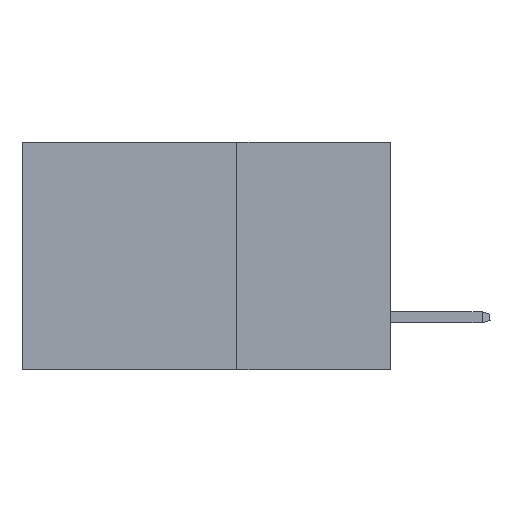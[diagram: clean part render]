
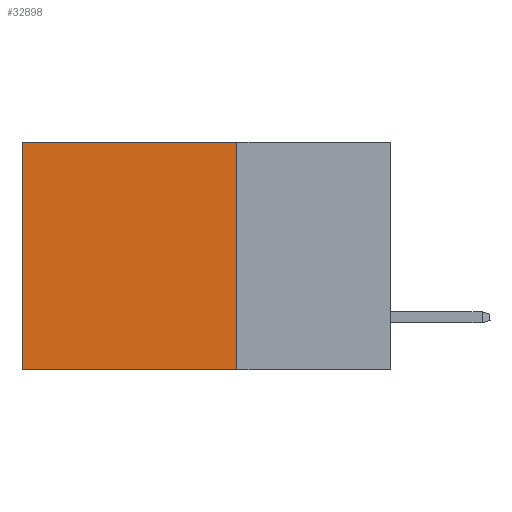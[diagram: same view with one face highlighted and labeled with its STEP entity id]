
A CAD part, left-side view. The second image highlights one B-rep face of the part: STEP entity #32898.
In plain terms, the highlighted planar face has unit normal (-1, 0, 0).
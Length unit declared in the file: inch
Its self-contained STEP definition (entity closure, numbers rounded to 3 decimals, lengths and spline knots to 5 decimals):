
#19 = VECTOR ( 'NONE', #25891, 39.37008 ) ;
#366 = CARTESIAN_POINT ( 'NONE',  ( 0.2875, 0.25, 0. ) ) ;
#2155 = LINE ( 'NONE', #31496, #19 ) ;
#2447 = FACE_OUTER_BOUND ( 'NONE', #20198, .T. ) ;
#3144 = CARTESIAN_POINT ( 'NONE',  ( 0.2875, 0.25, 0. ) ) ;
#3159 = DIRECTION ( 'NONE',  ( 0., 0., -1. ) ) ;
#5150 = PLANE ( 'NONE',  #31084 ) ;
#5556 = ORIENTED_EDGE ( 'NONE', *, *, #22146, .F. ) ;
#6188 = EDGE_CURVE ( 'NONE', #23111, #33666, #33103, .T. ) ;
#7851 = DIRECTION ( 'NONE',  ( 1., 0., 0. ) ) ;
#7975 = ORIENTED_EDGE ( 'NONE', *, *, #15313, .F. ) ;
#11665 = ORIENTED_EDGE ( 'NONE', *, *, #34053, .T. ) ;
#11965 = CARTESIAN_POINT ( 'NONE',  ( 0.2875, 0.25, -0.37 ) ) ;
#12003 = CARTESIAN_POINT ( 'NONE',  ( 0.2875, 0.25, -0.37 ) ) ;
#12150 = VERTEX_POINT ( 'NONE', #12003 ) ;
#13092 = VECTOR ( 'NONE', #34444, 39.37008 ) ;
#13201 = ORIENTED_EDGE ( 'NONE', *, *, #6188, .T. ) ;
#15313 = EDGE_CURVE ( 'NONE', #23111, #12150, #17719, .T. ) ;
#17719 = LINE ( 'NONE', #24684, #13092 ) ;
#18842 = LINE ( 'NONE', #11965, #31105 ) ;
#18974 = DIRECTION ( 'NONE',  ( 0., 1., 0. ) ) ;
#20198 = EDGE_LOOP ( 'NONE', ( #11665, #5556, #7975, #13201 ) ) ;
#22146 = EDGE_CURVE ( 'NONE', #12150, #24705, #18842, .T. ) ;
#23111 = VERTEX_POINT ( 'NONE', #366 ) ;
#23919 = CARTESIAN_POINT ( 'NONE',  ( 0.2875, 0.25, 0. ) ) ;
#24650 = VECTOR ( 'NONE', #18974, 39.37008 ) ;
#24684 = CARTESIAN_POINT ( 'NONE',  ( 0.2875, 0.25, 0. ) ) ;
#24705 = VERTEX_POINT ( 'NONE', #27690 ) ;
#25891 = DIRECTION ( 'NONE',  ( 0., 0., -1. ) ) ;
#27690 = CARTESIAN_POINT ( 'NONE',  ( 0.2875, 0.6, -0.37 ) ) ;
#30340 = CARTESIAN_POINT ( 'NONE',  ( 0.2875, 0.6, 0. ) ) ;
#31084 = AXIS2_PLACEMENT_3D ( 'NONE', #23919, #7851, #3159 ) ;
#31105 = VECTOR ( 'NONE', #33484, 39.37008 ) ;
#31496 = CARTESIAN_POINT ( 'NONE',  ( 0.2875, 0.6, 0. ) ) ;
#32898 = ADVANCED_FACE ( 'NONE', ( #2447 ), #5150, .F. ) ;
#33103 = LINE ( 'NONE', #3144, #24650 ) ;
#33484 = DIRECTION ( 'NONE',  ( 0., 1., 0. ) ) ;
#33666 = VERTEX_POINT ( 'NONE', #30340 ) ;
#34053 = EDGE_CURVE ( 'NONE', #33666, #24705, #2155, .T. ) ;
#34444 = DIRECTION ( 'NONE',  ( 0., 0., -1. ) ) ;
